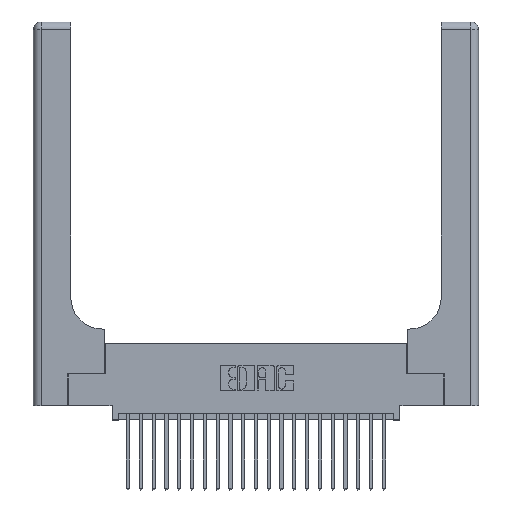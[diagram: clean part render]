
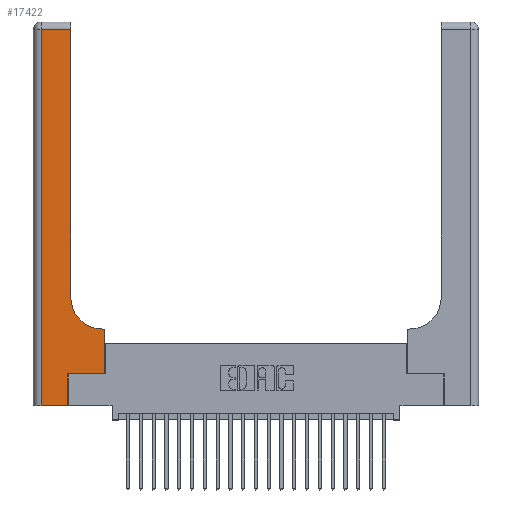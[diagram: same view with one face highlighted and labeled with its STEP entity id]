
A CAD part, top view. The second image highlights one B-rep face of the part: STEP entity #17422.
In plain terms, the highlighted planar face has unit normal (0, 0, 1).
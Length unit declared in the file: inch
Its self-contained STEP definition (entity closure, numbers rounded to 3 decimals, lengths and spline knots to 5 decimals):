
#694 = CARTESIAN_POINT ( 'NONE',  ( 0.2915, 0.85, 0.37 ) ) ;
#811 = CARTESIAN_POINT ( 'NONE',  ( 0.269, 0., 0.37 ) ) ;
#1138 = CARTESIAN_POINT ( 'NONE',  ( 0.5415, 0.6, 0.37 ) ) ;
#1482 = LINE ( 'NONE', #13644, #16185 ) ;
#1978 = LINE ( 'NONE', #14528, #11677 ) ;
#2369 = PLANE ( 'NONE',  #13449 ) ;
#3215 = CARTESIAN_POINT ( 'NONE',  ( 0.269, 0.25, 0.37 ) ) ;
#3768 = EDGE_CURVE ( 'NONE', #21819, #17540, #21192, .T. ) ;
#3958 = ORIENTED_EDGE ( 'NONE', *, *, #4424, .T. ) ;
#4264 = DIRECTION ( 'NONE',  ( 1., 0., 0. ) ) ;
#4424 = EDGE_CURVE ( 'NONE', #17540, #8144, #7687, .T. ) ;
#4429 = ORIENTED_EDGE ( 'NONE', *, *, #10920, .T. ) ;
#4660 = CARTESIAN_POINT ( 'NONE',  ( 0.06, 3., 0.37 ) ) ;
#4831 = LINE ( 'NONE', #4660, #24259 ) ;
#4998 = EDGE_LOOP ( 'NONE', ( #3958, #14997, #16169, #14704, #22323, #4429, #10762, #17782, #14003 ) ) ;
#5109 = DIRECTION ( 'NONE',  ( 0., 0., -1. ) ) ;
#5394 = DIRECTION ( 'NONE',  ( -1., 0., 0. ) ) ;
#6173 = CARTESIAN_POINT ( 'NONE',  ( 0.5585, 0.25, 0.37 ) ) ;
#6183 = LINE ( 'NONE', #19021, #16231 ) ;
#6486 = CARTESIAN_POINT ( 'NONE',  ( 0.5585, 0.6, 0.37 ) ) ;
#7053 = VECTOR ( 'NONE', #11162, 39.37008 ) ;
#7416 = VECTOR ( 'NONE', #5394, 39.37008 ) ;
#7687 = LINE ( 'NONE', #20442, #7053 ) ;
#7805 = DIRECTION ( 'NONE',  ( 0., 1., 0. ) ) ;
#7979 = VERTEX_POINT ( 'NONE', #6486 ) ;
#8138 = CARTESIAN_POINT ( 'NONE',  ( 0.06, 0., 0.37 ) ) ;
#8144 = VERTEX_POINT ( 'NONE', #20115 ) ;
#8281 = DIRECTION ( 'NONE',  ( 0., 0., -1. ) ) ;
#8960 = VECTOR ( 'NONE', #4264, 39.37008 ) ;
#8974 = DIRECTION ( 'NONE',  ( 0., 1., 0. ) ) ;
#9162 = EDGE_CURVE ( 'NONE', #12464, #7979, #1978, .T. ) ;
#9546 = LINE ( 'NONE', #22868, #8960 ) ;
#10201 = CARTESIAN_POINT ( 'NONE',  ( 0.06, 2.94, 0.37 ) ) ;
#10762 = ORIENTED_EDGE ( 'NONE', *, *, #9162, .T. ) ;
#10920 = EDGE_CURVE ( 'NONE', #18526, #12464, #18299, .T. ) ;
#11096 = CARTESIAN_POINT ( 'NONE',  ( 0.2915, 0.6, 0.37 ) ) ;
#11162 = DIRECTION ( 'NONE',  ( 0., 1., 0. ) ) ;
#11677 = VECTOR ( 'NONE', #8974, 39.37008 ) ;
#12331 = EDGE_CURVE ( 'NONE', #23407, #18526, #6183, .T. ) ;
#12340 = DIRECTION ( 'NONE',  ( 0., -1., 0. ) ) ;
#12464 = VERTEX_POINT ( 'NONE', #6173 ) ;
#12514 = VERTEX_POINT ( 'NONE', #10201 ) ;
#12879 = DIRECTION ( 'NONE',  ( 1., 0., 0. ) ) ;
#13234 = EDGE_CURVE ( 'NONE', #8144, #12514, #1482, .T. ) ;
#13344 = VECTOR ( 'NONE', #12879, 39.37008 ) ;
#13449 = AXIS2_PLACEMENT_3D ( 'NONE', #17616, #8281, #21359 ) ;
#13644 = CARTESIAN_POINT ( 'NONE',  ( 0., 2.94, 0.37 ) ) ;
#14003 = ORIENTED_EDGE ( 'NONE', *, *, #3768, .T. ) ;
#14528 = CARTESIAN_POINT ( 'NONE',  ( 0.5585, 0.25, 0.37 ) ) ;
#14679 = VERTEX_POINT ( 'NONE', #8138 ) ;
#14704 = ORIENTED_EDGE ( 'NONE', *, *, #17297, .T. ) ;
#14997 = ORIENTED_EDGE ( 'NONE', *, *, #13234, .T. ) ;
#15520 = DIRECTION ( 'NONE',  ( -1., 0., 0. ) ) ;
#15990 = FACE_OUTER_BOUND ( 'NONE', #4998, .T. ) ;
#16169 = ORIENTED_EDGE ( 'NONE', *, *, #21681, .T. ) ;
#16185 = VECTOR ( 'NONE', #15520, 39.37008 ) ;
#16231 = VECTOR ( 'NONE', #7805, 39.37008 ) ;
#16451 = CARTESIAN_POINT ( 'NONE',  ( 0.5415, 0.85, 0.37 ) ) ;
#16822 = LINE ( 'NONE', #11096, #7416 ) ;
#17297 = EDGE_CURVE ( 'NONE', #14679, #23407, #9546, .T. ) ;
#17422 = ADVANCED_FACE ( 'NONE', ( #15990 ), #2369, .F. ) ;
#17540 = VERTEX_POINT ( 'NONE', #694 ) ;
#17616 = CARTESIAN_POINT ( 'NONE',  ( 0., 3., 0.37 ) ) ;
#17782 = ORIENTED_EDGE ( 'NONE', *, *, #18800, .T. ) ;
#18299 = LINE ( 'NONE', #3215, #13344 ) ;
#18339 = DIRECTION ( 'NONE',  ( 1., 0., 0. ) ) ;
#18526 = VERTEX_POINT ( 'NONE', #24484 ) ;
#18800 = EDGE_CURVE ( 'NONE', #7979, #21819, #16822, .T. ) ;
#19021 = CARTESIAN_POINT ( 'NONE',  ( 0.269, 0., 0.37 ) ) ;
#20115 = CARTESIAN_POINT ( 'NONE',  ( 0.2915, 2.94, 0.37 ) ) ;
#20442 = CARTESIAN_POINT ( 'NONE',  ( 0.2915, 3., 0.37 ) ) ;
#21192 = CIRCLE ( 'NONE', #22443, 0.25 ) ;
#21359 = DIRECTION ( 'NONE',  ( -1., 0., 0. ) ) ;
#21681 = EDGE_CURVE ( 'NONE', #12514, #14679, #4831, .T. ) ;
#21819 = VERTEX_POINT ( 'NONE', #1138 ) ;
#22323 = ORIENTED_EDGE ( 'NONE', *, *, #12331, .T. ) ;
#22443 = AXIS2_PLACEMENT_3D ( 'NONE', #16451, #5109, #18339 ) ;
#22868 = CARTESIAN_POINT ( 'NONE',  ( 0., 0., 0.37 ) ) ;
#23407 = VERTEX_POINT ( 'NONE', #811 ) ;
#24259 = VECTOR ( 'NONE', #12340, 39.37008 ) ;
#24484 = CARTESIAN_POINT ( 'NONE',  ( 0.269, 0.25, 0.37 ) ) ;
